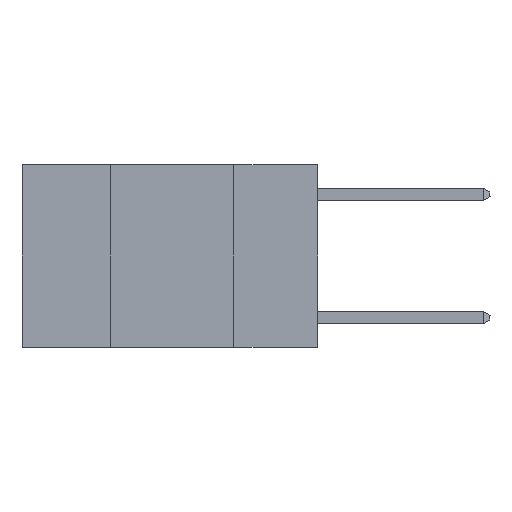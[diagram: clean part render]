
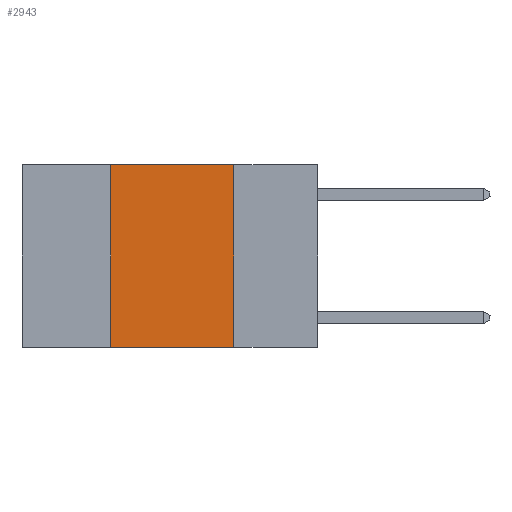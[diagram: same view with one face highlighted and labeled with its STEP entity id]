
A CAD part, left-side view. The second image highlights one B-rep face of the part: STEP entity #2943.
In plain terms, the highlighted planar face has unit normal (-1, 0, 0).
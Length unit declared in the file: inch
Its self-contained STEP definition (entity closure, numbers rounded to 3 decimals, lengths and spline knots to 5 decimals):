
#198 = CARTESIAN_POINT ( 'NONE',  ( 0., 0.42, -0.37 ) ) ;
#606 = AXIS2_PLACEMENT_3D ( 'NONE', #9421, #5718, #880 ) ;
#639 = DIRECTION ( 'NONE',  ( 0., -1., 0. ) ) ;
#789 = CARTESIAN_POINT ( 'NONE',  ( 0., 0.17, 0. ) ) ;
#841 = ORIENTED_EDGE ( 'NONE', *, *, #7680, .T. ) ;
#880 = DIRECTION ( 'NONE',  ( 0., 0., -1. ) ) ;
#1696 = DIRECTION ( 'NONE',  ( 0., 0., -1. ) ) ;
#2027 = CARTESIAN_POINT ( 'NONE',  ( 0., 0.17, -0.37 ) ) ;
#2943 = ADVANCED_FACE ( 'NONE', ( #12007 ), #9732, .F. ) ;
#3371 = VECTOR ( 'NONE', #639, 39.37008 ) ;
#4019 = EDGE_LOOP ( 'NONE', ( #4989, #13899, #11520, #841 ) ) ;
#4692 = VERTEX_POINT ( 'NONE', #789 ) ;
#4891 = DIRECTION ( 'NONE',  ( 0., 0., 1. ) ) ;
#4989 = ORIENTED_EDGE ( 'NONE', *, *, #7597, .F. ) ;
#5184 = VECTOR ( 'NONE', #11309, 39.37008 ) ;
#5206 = CARTESIAN_POINT ( 'NONE',  ( 0., 0.6, 0. ) ) ;
#5718 = DIRECTION ( 'NONE',  ( 1., 0., 0. ) ) ;
#5781 = VERTEX_POINT ( 'NONE', #2027 ) ;
#7197 = LINE ( 'NONE', #12075, #3371 ) ;
#7597 = EDGE_CURVE ( 'NONE', #4692, #5781, #14159, .T. ) ;
#7680 = EDGE_CURVE ( 'NONE', #12780, #5781, #7197, .T. ) ;
#8397 = VECTOR ( 'NONE', #4891, 39.37008 ) ;
#8703 = VERTEX_POINT ( 'NONE', #8856 ) ;
#8856 = CARTESIAN_POINT ( 'NONE',  ( 0., 0.42, 0. ) ) ;
#8899 = LINE ( 'NONE', #5206, #5184 ) ;
#9332 = EDGE_CURVE ( 'NONE', #12780, #8703, #9725, .T. ) ;
#9421 = CARTESIAN_POINT ( 'NONE',  ( 0., 0.6, 0. ) ) ;
#9725 = LINE ( 'NONE', #14472, #8397 ) ;
#9732 = PLANE ( 'NONE',  #606 ) ;
#11296 = EDGE_CURVE ( 'NONE', #8703, #4692, #8899, .T. ) ;
#11309 = DIRECTION ( 'NONE',  ( 0., -1., 0. ) ) ;
#11520 = ORIENTED_EDGE ( 'NONE', *, *, #9332, .F. ) ;
#11585 = CARTESIAN_POINT ( 'NONE',  ( 0., 0.17, 0. ) ) ;
#12007 = FACE_OUTER_BOUND ( 'NONE', #4019, .T. ) ;
#12075 = CARTESIAN_POINT ( 'NONE',  ( 0., 0.6, -0.37 ) ) ;
#12780 = VERTEX_POINT ( 'NONE', #198 ) ;
#13214 = VECTOR ( 'NONE', #1696, 39.37008 ) ;
#13899 = ORIENTED_EDGE ( 'NONE', *, *, #11296, .F. ) ;
#14159 = LINE ( 'NONE', #11585, #13214 ) ;
#14472 = CARTESIAN_POINT ( 'NONE',  ( 0., 0.42, 0. ) ) ;
